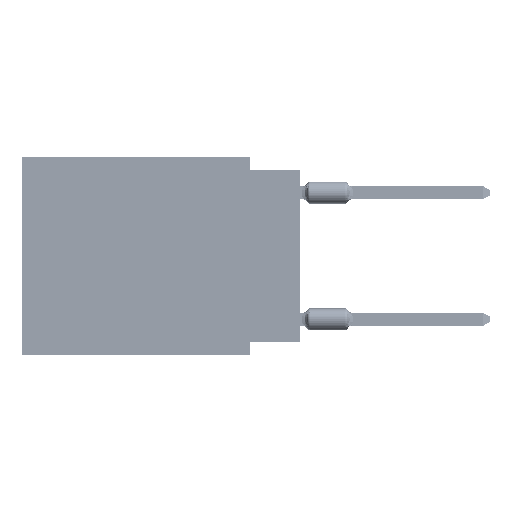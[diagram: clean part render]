
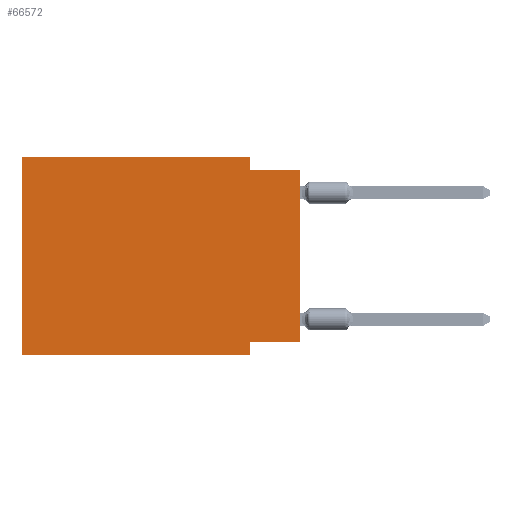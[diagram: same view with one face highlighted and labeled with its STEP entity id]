
A CAD part, left-side view. The second image highlights one B-rep face of the part: STEP entity #66572.
In plain terms, the highlighted planar face has unit normal (-1, 0, 0).
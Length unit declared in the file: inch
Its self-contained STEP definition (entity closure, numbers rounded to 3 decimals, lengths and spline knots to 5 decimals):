
#2744 = LINE ( 'NONE', #16205, #57286 ) ;
#3351 = CARTESIAN_POINT ( 'NONE',  ( 0., 0., -0.365 ) ) ;
#6168 = DIRECTION ( 'NONE',  ( 0., -1., 0. ) ) ;
#6473 = VECTOR ( 'NONE', #85056, 39.37008 ) ;
#10968 = DIRECTION ( 'NONE',  ( 0., 0., 1. ) ) ;
#12892 = CARTESIAN_POINT ( 'NONE',  ( 0., 0.55, -0.39 ) ) ;
#13419 = VECTOR ( 'NONE', #17906, 39.37008 ) ;
#16205 = CARTESIAN_POINT ( 'NONE',  ( 0., 0.55, 0. ) ) ;
#17906 = DIRECTION ( 'NONE',  ( 0., -1., 0. ) ) ;
#19183 = CARTESIAN_POINT ( 'NONE',  ( 0., 0., -0.025 ) ) ;
#19859 = DIRECTION ( 'NONE',  ( 0., 0., -1. ) ) ;
#25103 = LINE ( 'NONE', #51172, #6473 ) ;
#26753 = CARTESIAN_POINT ( 'NONE',  ( 0., 0.55, 0. ) ) ;
#27048 = VERTEX_POINT ( 'NONE', #55216 ) ;
#31306 = CARTESIAN_POINT ( 'NONE',  ( 0., 0., -0.025 ) ) ;
#31493 = DIRECTION ( 'NONE',  ( 0., 0., 1. ) ) ;
#31599 = CARTESIAN_POINT ( 'NONE',  ( 0., 0.1, -0.39 ) ) ;
#31716 = ORIENTED_EDGE ( 'NONE', *, *, #77964, .F. ) ;
#32469 = PLANE ( 'NONE',  #65019 ) ;
#32491 = CARTESIAN_POINT ( 'NONE',  ( 0., 0.1, -0.365 ) ) ;
#33109 = EDGE_CURVE ( 'NONE', #85092, #78566, #65697, .T. ) ;
#38853 = ORIENTED_EDGE ( 'NONE', *, *, #50340, .T. ) ;
#43068 = VECTOR ( 'NONE', #31493, 39.37008 ) ;
#44942 = EDGE_CURVE ( 'NONE', #85168, #85092, #2744, .T. ) ;
#45094 = EDGE_CURVE ( 'NONE', #76434, #46780, #73808, .T. ) ;
#45875 = EDGE_CURVE ( 'NONE', #81651, #51752, #73195, .T. ) ;
#46118 = ORIENTED_EDGE ( 'NONE', *, *, #33109, .F. ) ;
#46780 = VERTEX_POINT ( 'NONE', #31306 ) ;
#46792 = CARTESIAN_POINT ( 'NONE',  ( 0., 0.55, 0. ) ) ;
#47027 = ORIENTED_EDGE ( 'NONE', *, *, #45875, .F. ) ;
#48945 = VECTOR ( 'NONE', #6168, 39.37008 ) ;
#49330 = VECTOR ( 'NONE', #71190, 39.37008 ) ;
#49654 = CARTESIAN_POINT ( 'NONE',  ( 0., 0.1, 0. ) ) ;
#50340 = EDGE_CURVE ( 'NONE', #81651, #46780, #58449, .T. ) ;
#51172 = CARTESIAN_POINT ( 'NONE',  ( 0., 0.55, -0.39 ) ) ;
#51752 = VERTEX_POINT ( 'NONE', #32491 ) ;
#52024 = DIRECTION ( 'NONE',  ( 1., 0., 0. ) ) ;
#52756 = DIRECTION ( 'NONE',  ( 0., 1., 0. ) ) ;
#53684 = ORIENTED_EDGE ( 'NONE', *, *, #45094, .F. ) ;
#55216 = CARTESIAN_POINT ( 'NONE',  ( 0., 0.1, -0.39 ) ) ;
#56739 = CARTESIAN_POINT ( 'NONE',  ( 0., 0., 0. ) ) ;
#57286 = VECTOR ( 'NONE', #10968, 39.37008 ) ;
#58449 = LINE ( 'NONE', #56739, #43068 ) ;
#58551 = FACE_OUTER_BOUND ( 'NONE', #67494, .T. ) ;
#59284 = CARTESIAN_POINT ( 'NONE',  ( 0., 0., -0.365 ) ) ;
#59831 = LINE ( 'NONE', #74144, #78726 ) ;
#63753 = CARTESIAN_POINT ( 'NONE',  ( 0., 0.1, -0.025 ) ) ;
#64033 = EDGE_CURVE ( 'NONE', #85168, #27048, #25103, .T. ) ;
#65019 = AXIS2_PLACEMENT_3D ( 'NONE', #46792, #52024, #19859 ) ;
#65518 = LINE ( 'NONE', #31599, #49330 ) ;
#65697 = LINE ( 'NONE', #77867, #13419 ) ;
#66572 = ADVANCED_FACE ( 'NONE', ( #58551 ), #32469, .F. ) ;
#67494 = EDGE_LOOP ( 'NONE', ( #38853, #53684, #80160, #46118, #72567, #71991, #31716, #47027 ) ) ;
#71190 = DIRECTION ( 'NONE',  ( 0., 0., -1. ) ) ;
#71991 = ORIENTED_EDGE ( 'NONE', *, *, #64033, .T. ) ;
#72567 = ORIENTED_EDGE ( 'NONE', *, *, #44942, .F. ) ;
#73195 = LINE ( 'NONE', #59284, #76816 ) ;
#73808 = LINE ( 'NONE', #19183, #48945 ) ;
#74144 = CARTESIAN_POINT ( 'NONE',  ( 0., 0.1, 0. ) ) ;
#76434 = VERTEX_POINT ( 'NONE', #63753 ) ;
#76816 = VECTOR ( 'NONE', #52756, 39.37008 ) ;
#77867 = CARTESIAN_POINT ( 'NONE',  ( 0., 0.55, 0. ) ) ;
#77964 = EDGE_CURVE ( 'NONE', #51752, #27048, #65518, .T. ) ;
#78566 = VERTEX_POINT ( 'NONE', #49654 ) ;
#78726 = VECTOR ( 'NONE', #81078, 39.37008 ) ;
#80160 = ORIENTED_EDGE ( 'NONE', *, *, #82165, .F. ) ;
#81078 = DIRECTION ( 'NONE',  ( 0., 0., -1. ) ) ;
#81651 = VERTEX_POINT ( 'NONE', #3351 ) ;
#82165 = EDGE_CURVE ( 'NONE', #78566, #76434, #59831, .T. ) ;
#85056 = DIRECTION ( 'NONE',  ( 0., -1., 0. ) ) ;
#85092 = VERTEX_POINT ( 'NONE', #26753 ) ;
#85168 = VERTEX_POINT ( 'NONE', #12892 ) ;
